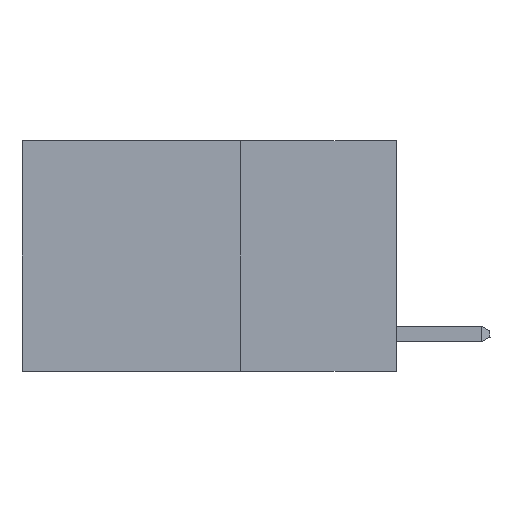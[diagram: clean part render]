
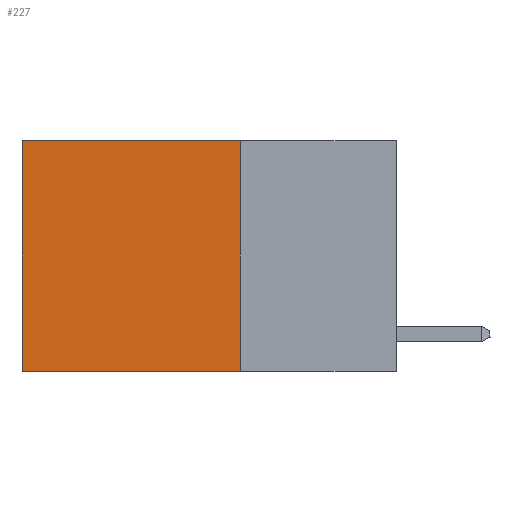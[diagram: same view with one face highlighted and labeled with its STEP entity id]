
A CAD part, left-side view. The second image highlights one B-rep face of the part: STEP entity #227.
In plain terms, the highlighted planar face has unit normal (-1, 0, 0).
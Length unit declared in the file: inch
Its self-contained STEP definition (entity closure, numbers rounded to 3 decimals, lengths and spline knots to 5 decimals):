
#227 = ADVANCED_FACE ( 'NONE', ( #6347 ), #13476, .F. ) ;
#656 = CARTESIAN_POINT ( 'NONE',  ( 0.2625, 0.25, 0. ) ) ;
#694 = VERTEX_POINT ( 'NONE', #13289 ) ;
#862 = VECTOR ( 'NONE', #13160, 39.37008 ) ;
#991 = DIRECTION ( 'NONE',  ( 1., 0., 0. ) ) ;
#3473 = EDGE_CURVE ( 'NONE', #7238, #9888, #3535, .T. ) ;
#3535 = LINE ( 'NONE', #13844, #24043 ) ;
#3920 = ORIENTED_EDGE ( 'NONE', *, *, #7537, .F. ) ;
#4637 = EDGE_CURVE ( 'NONE', #9888, #694, #17376, .T. ) ;
#5273 = DIRECTION ( 'NONE',  ( 0., 0., -1. ) ) ;
#5285 = AXIS2_PLACEMENT_3D ( 'NONE', #9338, #991, #15491 ) ;
#6347 = FACE_OUTER_BOUND ( 'NONE', #18550, .T. ) ;
#7238 = VERTEX_POINT ( 'NONE', #25768 ) ;
#7537 = EDGE_CURVE ( 'NONE', #8076, #694, #21785, .T. ) ;
#8076 = VERTEX_POINT ( 'NONE', #22488 ) ;
#9338 = CARTESIAN_POINT ( 'NONE',  ( 0.2625, 0.25, 0. ) ) ;
#9888 = VERTEX_POINT ( 'NONE', #20027 ) ;
#10182 = ORIENTED_EDGE ( 'NONE', *, *, #17794, .F. ) ;
#13160 = DIRECTION ( 'NONE',  ( 0., 0., -1. ) ) ;
#13289 = CARTESIAN_POINT ( 'NONE',  ( 0.2625, 0.6, -0.37 ) ) ;
#13476 = PLANE ( 'NONE',  #5285 ) ;
#13844 = CARTESIAN_POINT ( 'NONE',  ( 0.2625, 0.25, 0. ) ) ;
#14391 = ORIENTED_EDGE ( 'NONE', *, *, #4637, .T. ) ;
#15491 = DIRECTION ( 'NONE',  ( 0., 0., -1. ) ) ;
#15848 = DIRECTION ( 'NONE',  ( 0., 1., 0. ) ) ;
#16422 = VECTOR ( 'NONE', #24633, 39.37008 ) ;
#16506 = CARTESIAN_POINT ( 'NONE',  ( 0.2625, 0.25, -0.37 ) ) ;
#17376 = LINE ( 'NONE', #19679, #22737 ) ;
#17794 = EDGE_CURVE ( 'NONE', #7238, #8076, #22728, .T. ) ;
#18550 = EDGE_LOOP ( 'NONE', ( #14391, #3920, #10182, #21792 ) ) ;
#19679 = CARTESIAN_POINT ( 'NONE',  ( 0.2625, 0.6, 0. ) ) ;
#20027 = CARTESIAN_POINT ( 'NONE',  ( 0.2625, 0.6, 0. ) ) ;
#21785 = LINE ( 'NONE', #16506, #16422 ) ;
#21792 = ORIENTED_EDGE ( 'NONE', *, *, #3473, .T. ) ;
#22488 = CARTESIAN_POINT ( 'NONE',  ( 0.2625, 0.25, -0.37 ) ) ;
#22728 = LINE ( 'NONE', #656, #862 ) ;
#22737 = VECTOR ( 'NONE', #5273, 39.37008 ) ;
#24043 = VECTOR ( 'NONE', #15848, 39.37008 ) ;
#24633 = DIRECTION ( 'NONE',  ( 0., 1., 0. ) ) ;
#25768 = CARTESIAN_POINT ( 'NONE',  ( 0.2625, 0.25, 0. ) ) ;
